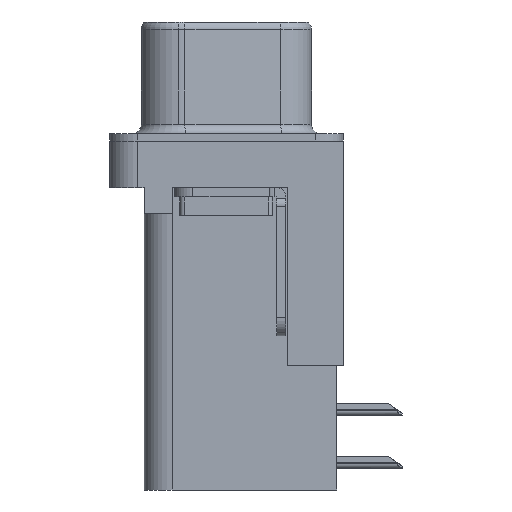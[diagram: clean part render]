
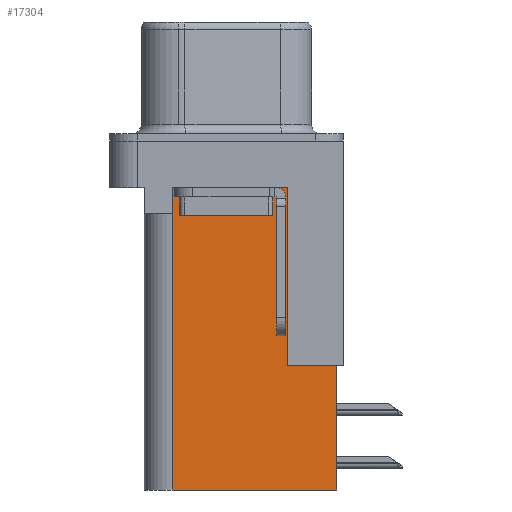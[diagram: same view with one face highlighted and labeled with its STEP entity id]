
A CAD part, left-side view. The second image highlights one B-rep face of the part: STEP entity #17304.
In plain terms, the highlighted planar face has unit normal (-1, 0, 0).
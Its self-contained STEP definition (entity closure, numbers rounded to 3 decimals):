
#52 = LINE ( 'NONE', #3885, #18296 ) ;
#210 = VERTEX_POINT ( 'NONE', #20564 ) ;
#316 = DIRECTION ( 'NONE',  ( 0., 0., 1. ) ) ;
#583 = EDGE_LOOP ( 'NONE', ( #13051, #16881, #21097, #22587, #9052, #3514, #18892, #12643 ) ) ;
#1011 = LINE ( 'NONE', #16186, #14565 ) ;
#1346 = DIRECTION ( 'NONE',  ( 0., 1., 0. ) ) ;
#1972 = VECTOR ( 'NONE', #9798, 1000. ) ;
#2777 = DIRECTION ( 'NONE',  ( 0., 1., 0. ) ) ;
#2878 = DIRECTION ( 'NONE',  ( 0., 0., -1. ) ) ;
#3135 = VECTOR ( 'NONE', #1346, 1000. ) ;
#3262 = VECTOR ( 'NONE', #10849, 1000. ) ;
#3514 = ORIENTED_EDGE ( 'NONE', *, *, #10268, .F. ) ;
#3885 = CARTESIAN_POINT ( 'NONE',  ( 3.7, -3.295, -18.76 ) ) ;
#4094 = VERTEX_POINT ( 'NONE', #7949 ) ;
#4205 = LINE ( 'NONE', #20037, #4759 ) ;
#4759 = VECTOR ( 'NONE', #9523, 1000. ) ;
#6090 = VECTOR ( 'NONE', #2777, 1000. ) ;
#6346 = CARTESIAN_POINT ( 'NONE',  ( 3.7, 2.925, -3.9 ) ) ;
#6641 = LINE ( 'NONE', #7961, #1972 ) ;
#7165 = EDGE_CURVE ( 'NONE', #210, #13764, #21892, .T. ) ;
#7192 = CARTESIAN_POINT ( 'NONE',  ( 3.7, -3.295, -12.05 ) ) ;
#7587 = CARTESIAN_POINT ( 'NONE',  ( 3.7, -5.925, -18.76 ) ) ;
#7949 = CARTESIAN_POINT ( 'NONE',  ( 3.7, -3.295, -2.5 ) ) ;
#7961 = CARTESIAN_POINT ( 'NONE',  ( 3.7, -6.295, -12.05 ) ) ;
#8280 = LINE ( 'NONE', #11948, #3135 ) ;
#8583 = EDGE_CURVE ( 'NONE', #21818, #210, #52, .T. ) ;
#9026 = CARTESIAN_POINT ( 'NONE',  ( 3.7, 2.925, -18.76 ) ) ;
#9052 = ORIENTED_EDGE ( 'NONE', *, *, #8583, .F. ) ;
#9467 = VERTEX_POINT ( 'NONE', #21692 ) ;
#9523 = DIRECTION ( 'NONE',  ( 0., 0., -1. ) ) ;
#9798 = DIRECTION ( 'NONE',  ( 0., 1., 0. ) ) ;
#10259 = DIRECTION ( 'NONE',  ( 1., 0., 0. ) ) ;
#10268 = EDGE_CURVE ( 'NONE', #9467, #21818, #21009, .T. ) ;
#10584 = VERTEX_POINT ( 'NONE', #21699 ) ;
#10849 = DIRECTION ( 'NONE',  ( 0., 0., 1. ) ) ;
#11466 = EDGE_CURVE ( 'NONE', #9467, #22169, #6641, .T. ) ;
#11646 = CARTESIAN_POINT ( 'NONE',  ( 3.7, -5.925, -2. ) ) ;
#11691 = VECTOR ( 'NONE', #2878, 1000. ) ;
#11948 = CARTESIAN_POINT ( 'NONE',  ( 3.7, 0., -3.9 ) ) ;
#12463 = EDGE_CURVE ( 'NONE', #4094, #14506, #15984, .T. ) ;
#12643 = ORIENTED_EDGE ( 'NONE', *, *, #14120, .T. ) ;
#13051 = ORIENTED_EDGE ( 'NONE', *, *, #12463, .T. ) ;
#13651 = FACE_OUTER_BOUND ( 'NONE', #583, .T. ) ;
#13764 = VERTEX_POINT ( 'NONE', #6346 ) ;
#14120 = EDGE_CURVE ( 'NONE', #22169, #4094, #1011, .T. ) ;
#14412 = DIRECTION ( 'NONE',  ( 0., 1., 0. ) ) ;
#14506 = VERTEX_POINT ( 'NONE', #15230 ) ;
#14565 = VECTOR ( 'NONE', #316, 1000. ) ;
#15230 = CARTESIAN_POINT ( 'NONE',  ( 3.7, 2.895, -2.5 ) ) ;
#15984 = LINE ( 'NONE', #21997, #6090 ) ;
#16186 = CARTESIAN_POINT ( 'NONE',  ( 3.7, -3.295, -18.76 ) ) ;
#16881 = ORIENTED_EDGE ( 'NONE', *, *, #22359, .T. ) ;
#17304 = ADVANCED_FACE ( 'NONE', ( #13651 ), #20774, .F. ) ;
#18296 = VECTOR ( 'NONE', #14412, 1000. ) ;
#18892 = ORIENTED_EDGE ( 'NONE', *, *, #11466, .T. ) ;
#20037 = CARTESIAN_POINT ( 'NONE',  ( 3.7, 2.895, -3.9 ) ) ;
#20564 = CARTESIAN_POINT ( 'NONE',  ( 3.7, 2.925, -18.76 ) ) ;
#20774 = PLANE ( 'NONE',  #21884 ) ;
#21009 = LINE ( 'NONE', #11646, #11691 ) ;
#21097 = ORIENTED_EDGE ( 'NONE', *, *, #21366, .T. ) ;
#21366 = EDGE_CURVE ( 'NONE', #10584, #13764, #8280, .T. ) ;
#21692 = CARTESIAN_POINT ( 'NONE',  ( 3.7, -5.925, -12.05 ) ) ;
#21699 = CARTESIAN_POINT ( 'NONE',  ( 3.7, 2.895, -3.9 ) ) ;
#21818 = VERTEX_POINT ( 'NONE', #7587 ) ;
#21884 = AXIS2_PLACEMENT_3D ( 'NONE', #22425, #10259, #22486 ) ;
#21892 = LINE ( 'NONE', #9026, #3262 ) ;
#21997 = CARTESIAN_POINT ( 'NONE',  ( 3.7, -3.295, -2.5 ) ) ;
#22169 = VERTEX_POINT ( 'NONE', #7192 ) ;
#22359 = EDGE_CURVE ( 'NONE', #14506, #10584, #4205, .T. ) ;
#22425 = CARTESIAN_POINT ( 'NONE',  ( 3.7, -3.295, -18.76 ) ) ;
#22486 = DIRECTION ( 'NONE',  ( 0., 1., 0. ) ) ;
#22587 = ORIENTED_EDGE ( 'NONE', *, *, #7165, .F. ) ;
